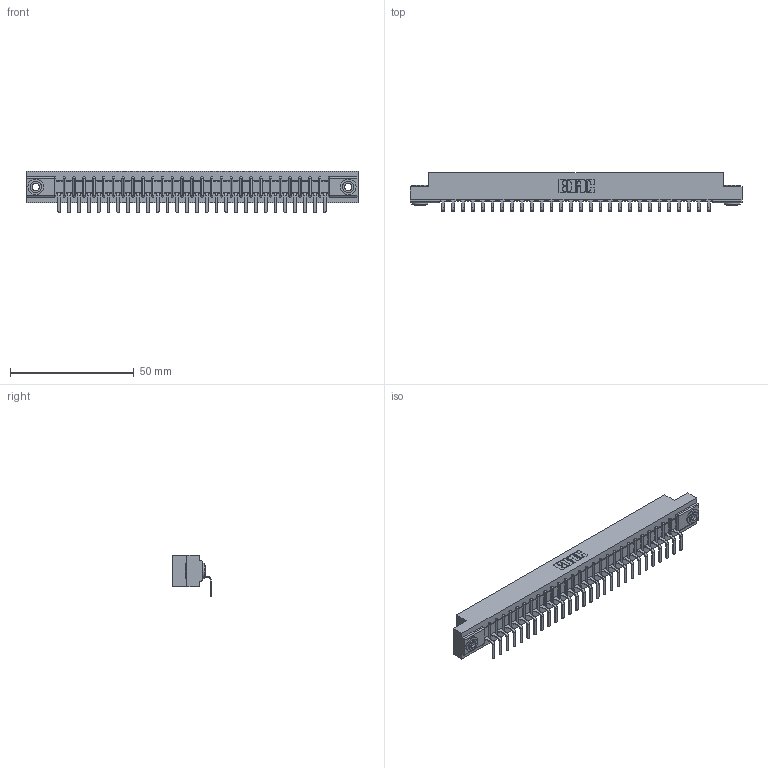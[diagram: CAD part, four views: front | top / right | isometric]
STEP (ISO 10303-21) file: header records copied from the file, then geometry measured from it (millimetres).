
FILE_DESCRIPTION (( 'STEP AP203' ), '1' );
FILE_NAME ('307-028-559-103.STEP', '2019-09-04T16:43:01', ( '' ), ( '' ), 'SwSTEP 2.0', 'SolidWorks 2016', '' );
FILE_SCHEMA (( 'CONFIG_CONTROL_DESIGN' ));
Length unit declared in the file: inch
Products named in the file (4): 307 Part_.156 Dia Mounting Holes; 307-028-559-103; 307-290-001_558 559 - 1 (Single); 345-250-002_345-250-002-102
Assembly tree (31 placements, depth 2):
  307-028-559-103
    307 Part_.156 Dia Mounting Holes
    307-290-001_558 559 - 1 (Single)  x28
    345-250-002_345-250-002-102  x2
Bounding box: 133.96 x 15.46 x 16.8 mm (x, y, z)
Volume: 13862.3 mm3; surface area: 14968.3 mm2
Topology: 31 solids, 31 shells, 1879 faces, 5307 edges, 3418 vertices
Faces by surface type: plane 1186, cylinder 627, sphere 58, cone 8
Entity records: 26899 total; most frequent: CARTESIAN_POINT 4505, ORIENTED_EDGE 4482, DIRECTION 4405, EDGE_CURVE 2241, VECTOR 1705, LINE 1705, VERTEX_POINT 1450, AXIS2_PLACEMENT_3D 1350
